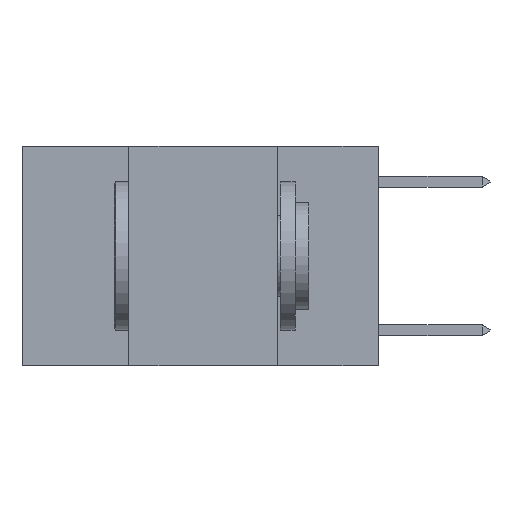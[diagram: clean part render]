
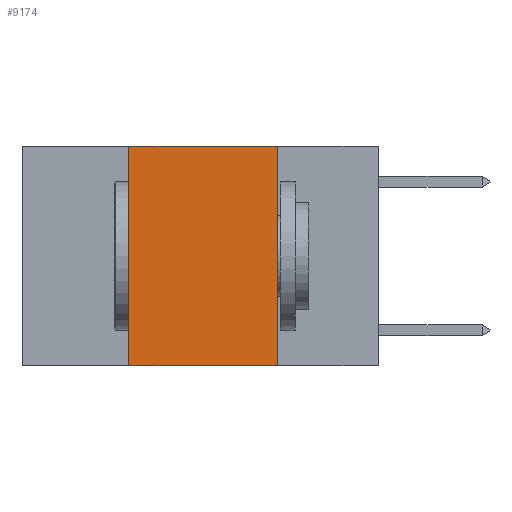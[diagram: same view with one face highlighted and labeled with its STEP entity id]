
A CAD part, left-side view. The second image highlights one B-rep face of the part: STEP entity #9174.
In plain terms, the highlighted planar face has unit normal (-1, 0, 0).
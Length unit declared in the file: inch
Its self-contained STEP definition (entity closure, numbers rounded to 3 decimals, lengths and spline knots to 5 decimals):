
#426 = EDGE_CURVE ( 'NONE', #9301, #7364, #11126, .T. ) ;
#593 = LINE ( 'NONE', #10339, #1776 ) ;
#760 = AXIS2_PLACEMENT_3D ( 'NONE', #9568, #1479, #7800 ) ;
#1180 = ORIENTED_EDGE ( 'NONE', *, *, #426, .F. ) ;
#1213 = CARTESIAN_POINT ( 'NONE',  ( 0., 0.17, 0. ) ) ;
#1479 = DIRECTION ( 'NONE',  ( 1., 0., 0. ) ) ;
#1488 = VECTOR ( 'NONE', #3395, 39.37008 ) ;
#1776 = VECTOR ( 'NONE', #5901, 39.37008 ) ;
#2880 = EDGE_LOOP ( 'NONE', ( #1180, #3285, #8885, #4816 ) ) ;
#3285 = ORIENTED_EDGE ( 'NONE', *, *, #7806, .F. ) ;
#3336 = EDGE_CURVE ( 'NONE', #5025, #8940, #4253, .T. ) ;
#3395 = DIRECTION ( 'NONE',  ( 0., 0., 1. ) ) ;
#4253 = LINE ( 'NONE', #7861, #1488 ) ;
#4816 = ORIENTED_EDGE ( 'NONE', *, *, #5250, .T. ) ;
#5025 = VERTEX_POINT ( 'NONE', #11327 ) ;
#5250 = EDGE_CURVE ( 'NONE', #5025, #7364, #6854, .T. ) ;
#5901 = DIRECTION ( 'NONE',  ( 0., -1., 0. ) ) ;
#5958 = PLANE ( 'NONE',  #760 ) ;
#6076 = CARTESIAN_POINT ( 'NONE',  ( 0., 0.17, 0. ) ) ;
#6092 = CARTESIAN_POINT ( 'NONE',  ( 0., 0.6, -0.37 ) ) ;
#6854 = LINE ( 'NONE', #6092, #7684 ) ;
#6910 = DIRECTION ( 'NONE',  ( 0., -1., 0. ) ) ;
#7364 = VERTEX_POINT ( 'NONE', #7756 ) ;
#7684 = VECTOR ( 'NONE', #6910, 39.37008 ) ;
#7756 = CARTESIAN_POINT ( 'NONE',  ( 0., 0.17, -0.37 ) ) ;
#7800 = DIRECTION ( 'NONE',  ( 0., 0., -1. ) ) ;
#7806 = EDGE_CURVE ( 'NONE', #8940, #9301, #593, .T. ) ;
#7861 = CARTESIAN_POINT ( 'NONE',  ( 0., 0.42, 0. ) ) ;
#8449 = DIRECTION ( 'NONE',  ( 0., 0., -1. ) ) ;
#8868 = CARTESIAN_POINT ( 'NONE',  ( 0., 0.42, 0. ) ) ;
#8885 = ORIENTED_EDGE ( 'NONE', *, *, #3336, .F. ) ;
#8940 = VERTEX_POINT ( 'NONE', #8868 ) ;
#9174 = ADVANCED_FACE ( 'NONE', ( #11337 ), #5958, .F. ) ;
#9301 = VERTEX_POINT ( 'NONE', #6076 ) ;
#9568 = CARTESIAN_POINT ( 'NONE',  ( 0., 0.6, 0. ) ) ;
#10339 = CARTESIAN_POINT ( 'NONE',  ( 0., 0.6, 0. ) ) ;
#11126 = LINE ( 'NONE', #1213, #11436 ) ;
#11327 = CARTESIAN_POINT ( 'NONE',  ( 0., 0.42, -0.37 ) ) ;
#11337 = FACE_OUTER_BOUND ( 'NONE', #2880, .T. ) ;
#11436 = VECTOR ( 'NONE', #8449, 39.37008 ) ;
